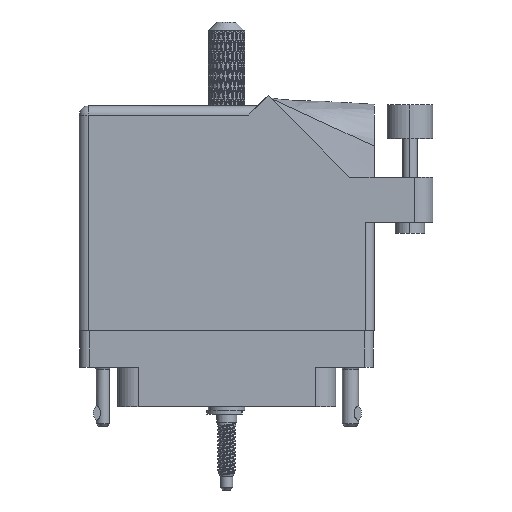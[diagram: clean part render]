
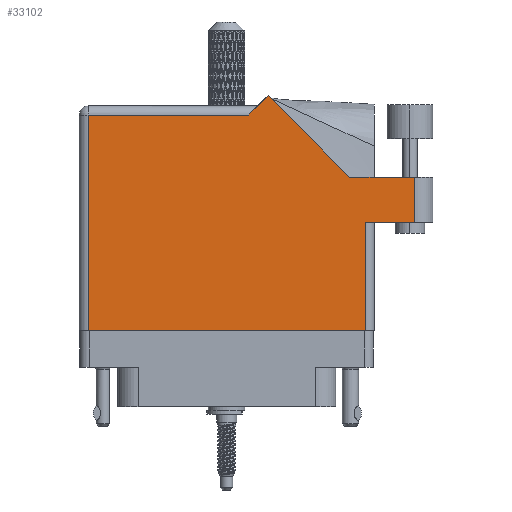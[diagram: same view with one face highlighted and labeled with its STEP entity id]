
A CAD part, front view. The second image highlights one B-rep face of the part: STEP entity #33102.
In plain terms, the highlighted face is planar.
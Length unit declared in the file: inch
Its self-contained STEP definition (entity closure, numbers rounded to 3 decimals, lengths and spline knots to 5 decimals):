
#559 = LINE ( 'NONE', #23286, #91846 ) ;
#3743 = VECTOR ( 'NONE', #67856, 39.37008 ) ;
#4225 = LINE ( 'NONE', #102249, #92844 ) ;
#4490 = ORIENTED_EDGE ( 'NONE', *, *, #20189, .T. ) ;
#5128 = LINE ( 'NONE', #84420, #3743 ) ;
#8700 = ORIENTED_EDGE ( 'NONE', *, *, #51930, .T. ) ;
#9289 = EDGE_CURVE ( 'NONE', #70792, #65086, #5128, .T. ) ;
#10093 = DIRECTION ( 'NONE',  ( -0.707, -0.707, 0. ) ) ;
#11786 = EDGE_CURVE ( 'NONE', #27834, #95193, #51742, .T. ) ;
#15096 = EDGE_CURVE ( 'NONE', #87524, #23420, #32722, .T. ) ;
#15336 = CARTESIAN_POINT ( 'NONE',  ( 0.28271, 1.50071, 0.455 ) ) ;
#16843 = CARTESIAN_POINT ( 'NONE',  ( -0.943, 1.368, 0.455 ) ) ;
#18147 = LINE ( 'NONE', #72400, #106724 ) ;
#18812 = DIRECTION ( 'NONE',  ( -1., 0., 0. ) ) ;
#20189 = EDGE_CURVE ( 'NONE', #75517, #96059, #110037, .T. ) ;
#23286 = CARTESIAN_POINT ( 'NONE',  ( 0.83942, 0.944, 0.455 ) ) ;
#23420 = VERTEX_POINT ( 'NONE', #61951 ) ;
#27834 = VERTEX_POINT ( 'NONE', #83154 ) ;
#28204 = VECTOR ( 'NONE', #10093, 39.37008 ) ;
#30408 = DIRECTION ( 'NONE',  ( 0., -1., 0. ) ) ;
#30572 = DIRECTION ( 'NONE',  ( 1., 0., 0. ) ) ;
#32057 = AXIS2_PLACEMENT_3D ( 'NONE', #72858, #39815, #82274 ) ;
#32722 = LINE ( 'NONE', #42796, #67553 ) ;
#33102 = ADVANCED_FACE ( 'NONE', ( #73376 ), #89849, .F. ) ;
#33540 = DIRECTION ( 'NONE',  ( 0., 1., 0. ) ) ;
#34931 = EDGE_CURVE ( 'NONE', #65086, #27834, #18147, .T. ) ;
#38328 = ORIENTED_EDGE ( 'NONE', *, *, #46383, .T. ) ;
#39815 = DIRECTION ( 'NONE',  ( 0., 0., -1. ) ) ;
#42342 = VECTOR ( 'NONE', #63747, 39.37008 ) ;
#42796 = CARTESIAN_POINT ( 'NONE',  ( 1.405, 0.944, 0.455 ) ) ;
#43182 = CARTESIAN_POINT ( 'NONE',  ( 1.28, 0.637, 0.455 ) ) ;
#46383 = EDGE_CURVE ( 'NONE', #23420, #62384, #559, .T. ) ;
#48079 = ORIENTED_EDGE ( 'NONE', *, *, #9289, .T. ) ;
#51742 = LINE ( 'NONE', #82099, #42342 ) ;
#51930 = EDGE_CURVE ( 'NONE', #95193, #75517, #4225, .T. ) ;
#55258 = ORIENTED_EDGE ( 'NONE', *, *, #15096, .T. ) ;
#58524 = ORIENTED_EDGE ( 'NONE', *, *, #11786, .T. ) ;
#61057 = EDGE_CURVE ( 'NONE', #62384, #70792, #73823, .T. ) ;
#61951 = CARTESIAN_POINT ( 'NONE',  ( 0.83942, 0.944, 0.455 ) ) ;
#62384 = VERTEX_POINT ( 'NONE', #15336 ) ;
#63747 = DIRECTION ( 'NONE',  ( 1., 0., 0. ) ) ;
#65086 = VERTEX_POINT ( 'NONE', #16843 ) ;
#65659 = CARTESIAN_POINT ( 'NONE',  ( 1.28, 0.944, 0.455 ) ) ;
#65740 = CARTESIAN_POINT ( 'NONE',  ( 0.15, 1.368, 0.455 ) ) ;
#65990 = DIRECTION ( 'NONE',  ( -0.707, 0.707, 0. ) ) ;
#67553 = VECTOR ( 'NONE', #18812, 39.37008 ) ;
#67856 = DIRECTION ( 'NONE',  ( -1., 0., 0. ) ) ;
#69034 = CARTESIAN_POINT ( 'NONE',  ( 1.28, 0.944, 0.455 ) ) ;
#70792 = VERTEX_POINT ( 'NONE', #65740 ) ;
#72400 = CARTESIAN_POINT ( 'NONE',  ( -0.943, -0.1, 0.455 ) ) ;
#72858 = CARTESIAN_POINT ( 'NONE',  ( -1.005, 1.43, 0.455 ) ) ;
#73376 = FACE_OUTER_BOUND ( 'NONE', #95255, .T. ) ;
#73823 = LINE ( 'NONE', #94523, #28204 ) ;
#74053 = CARTESIAN_POINT ( 'NONE',  ( 1.005, 0.637, 0.455 ) ) ;
#75517 = VERTEX_POINT ( 'NONE', #101880 ) ;
#76778 = LINE ( 'NONE', #69034, #84933 ) ;
#80657 = ORIENTED_EDGE ( 'NONE', *, *, #61057, .T. ) ;
#82099 = CARTESIAN_POINT ( 'NONE',  ( -1.005, -0.1, 0.455 ) ) ;
#82274 = DIRECTION ( 'NONE',  ( -1., 0., 0. ) ) ;
#83154 = CARTESIAN_POINT ( 'NONE',  ( -0.943, -0.1, 0.455 ) ) ;
#84420 = CARTESIAN_POINT ( 'NONE',  ( -1.005, 1.368, 0.455 ) ) ;
#84933 = VECTOR ( 'NONE', #96096, 39.37008 ) ;
#86976 = ORIENTED_EDGE ( 'NONE', *, *, #96099, .T. ) ;
#87524 = VERTEX_POINT ( 'NONE', #65659 ) ;
#89849 = PLANE ( 'NONE',  #32057 ) ;
#91846 = VECTOR ( 'NONE', #65990, 39.37008 ) ;
#91918 = CARTESIAN_POINT ( 'NONE',  ( 0.943, -0.1, 0.455 ) ) ;
#92844 = VECTOR ( 'NONE', #33540, 39.37008 ) ;
#94523 = CARTESIAN_POINT ( 'NONE',  ( 0.212, 1.43, 0.455 ) ) ;
#95193 = VERTEX_POINT ( 'NONE', #91918 ) ;
#95255 = EDGE_LOOP ( 'NONE', ( #4490, #86976, #55258, #38328, #80657, #48079, #101365, #58524, #8700 ) ) ;
#96059 = VERTEX_POINT ( 'NONE', #43182 ) ;
#96096 = DIRECTION ( 'NONE',  ( 0., 1., 0. ) ) ;
#96099 = EDGE_CURVE ( 'NONE', #96059, #87524, #76778, .T. ) ;
#101365 = ORIENTED_EDGE ( 'NONE', *, *, #34931, .T. ) ;
#101880 = CARTESIAN_POINT ( 'NONE',  ( 0.943, 0.637, 0.455 ) ) ;
#102249 = CARTESIAN_POINT ( 'NONE',  ( 0.943, 0.637, 0.455 ) ) ;
#103285 = VECTOR ( 'NONE', #30572, 39.37008 ) ;
#106724 = VECTOR ( 'NONE', #30408, 39.37008 ) ;
#110037 = LINE ( 'NONE', #74053, #103285 ) ;
